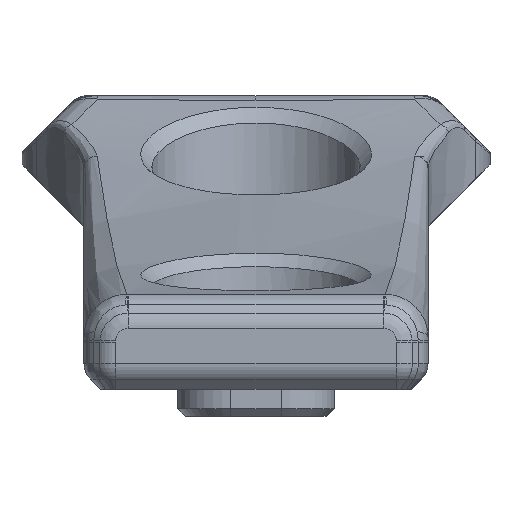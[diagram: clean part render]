
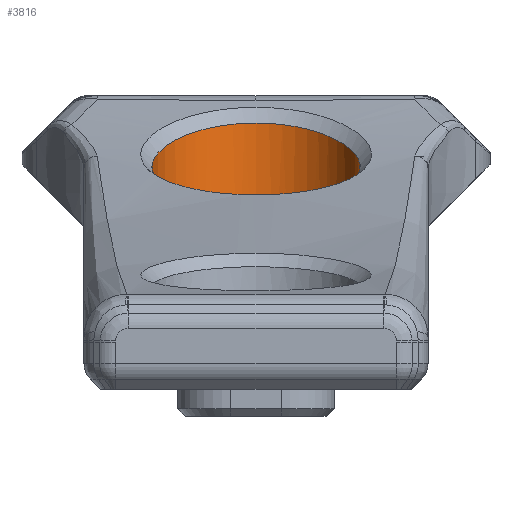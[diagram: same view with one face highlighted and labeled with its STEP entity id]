
A CAD part, front view. The second image highlights one B-rep face of the part: STEP entity #3816.
In plain terms, the highlighted cylindrical face has radius 4.65 mm (diameter 9.3 mm), a full revolution.
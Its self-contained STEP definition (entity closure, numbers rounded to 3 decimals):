
#304=CIRCLE('',#4113,4.65);
#429=FACE_OUTER_BOUND('',#678,.T.);
#678=EDGE_LOOP('',(#2908,#2909,#2910,#2911,#2912));
#931=LINE('',#6753,#1177);
#1177=VECTOR('',#4613,4.65);
#1433=B_SPLINE_CURVE_WITH_KNOTS('',3,(#6720,#6721,#6722,#6723,#6724,#6725,
#6726,#6727,#6728,#6729,#6730,#6731,#6732,#6733,#6734,#6735,#6736,#6737,
#6738,#6739),.UNSPECIFIED.,.F.,.F.,(4,1,1,1,1,1,1,1,1,1,1,1,1,1,1,1,1,4),
(0.,0.207,0.311,0.415,0.57,
0.622,0.829,0.968,1.244,1.313,
1.382,1.521,1.659,1.762,1.866,
2.022,2.073,2.155),.UNSPECIFIED.);
#1434=B_SPLINE_CURVE_WITH_KNOTS('',3,(#6740,#6741,#6742,#6743,#6744,#6745,
#6746,#6747,#6748,#6749),.UNSPECIFIED.,.F.,.F.,(4,1,1,1,1,1,1,4),(2.155,
2.281,2.488,2.566,2.592,2.696,
2.799,2.903),.UNSPECIFIED.);
#1711=VERTEX_POINT('',#6717);
#1712=VERTEX_POINT('',#6719);
#1713=VERTEX_POINT('',#6751);
#2141=EDGE_CURVE('',#1711,#1712,#1433,.T.);
#2142=EDGE_CURVE('',#1712,#1711,#1434,.T.);
#2143=EDGE_CURVE('',#1713,#1713,#304,.T.);
#2144=EDGE_CURVE('',#1713,#1712,#931,.T.);
#2908=ORIENTED_EDGE('',*,*,#2143,.T.);
#2909=ORIENTED_EDGE('',*,*,#2144,.T.);
#2910=ORIENTED_EDGE('',*,*,#2141,.F.);
#2911=ORIENTED_EDGE('',*,*,#2142,.F.);
#2912=ORIENTED_EDGE('',*,*,#2144,.F.);
#3699=CYLINDRICAL_SURFACE('',#4112,4.65);
#3816=ADVANCED_FACE('',(#429),#3699,.F.);
#4112=AXIS2_PLACEMENT_3D('',#6750,#4609,#4610);
#4113=AXIS2_PLACEMENT_3D('',#6752,#4611,#4612);
#4609=DIRECTION('center_axis',(0.,0.,1.));
#4610=DIRECTION('ref_axis',(1.,0.,0.));
#4611=DIRECTION('center_axis',(0.,0.,-1.));
#4612=DIRECTION('ref_axis',(1.,0.,0.));
#4613=DIRECTION('',(0.,0.,1.));
#6717=CARTESIAN_POINT('',(0.,38.65,11.102));
#6719=CARTESIAN_POINT('',(-4.651,33.998,9.158));
#6720=CARTESIAN_POINT('Ctrl Pts',(0.,38.65,11.102));
#6721=CARTESIAN_POINT('Ctrl Pts',(0.658,38.65,11.102));
#6722=CARTESIAN_POINT('Ctrl Pts',(1.717,38.423,10.996));
#6723=CARTESIAN_POINT('Ctrl Pts',(2.883,37.691,10.668));
#6724=CARTESIAN_POINT('Ctrl Pts',(3.701,36.904,10.325));
#6725=CARTESIAN_POINT('Ctrl Pts',(4.242,36.007,9.949));
#6726=CARTESIAN_POINT('Ctrl Pts',(4.657,34.705,9.426));
#6727=CARTESIAN_POINT('Ctrl Pts',(4.731,33.442,8.942));
#6728=CARTESIAN_POINT('Ctrl Pts',(4.041,31.371,8.202));
#6729=CARTESIAN_POINT('Ctrl Pts',(2.857,30.163,7.806));
#6730=CARTESIAN_POINT('Ctrl Pts',(1.461,29.563,7.614));
#6731=CARTESIAN_POINT('Ctrl Pts',(0.482,29.332,7.541));
#6732=CARTESIAN_POINT('Ctrl Pts',(-0.723,29.327,7.539));
#6733=CARTESIAN_POINT('Ctrl Pts',(-2.074,29.764,7.677));
#6734=CARTESIAN_POINT('Ctrl Pts',(-3.084,30.469,7.907));
#6735=CARTESIAN_POINT('Ctrl Pts',(-3.906,31.364,8.207));
#6736=CARTESIAN_POINT('Ctrl Pts',(-4.397,32.351,8.55));
#6737=CARTESIAN_POINT('Ctrl Pts',(-4.611,33.303,8.897));
#6738=CARTESIAN_POINT('Ctrl Pts',(-4.65,33.736,9.059));
#6739=CARTESIAN_POINT('Ctrl Pts',(-4.651,33.998,9.158));
#6740=CARTESIAN_POINT('Ctrl Pts',(-4.651,33.998,9.158));
#6741=CARTESIAN_POINT('Ctrl Pts',(-4.653,34.402,9.311));
#6742=CARTESIAN_POINT('Ctrl Pts',(-4.516,35.456,9.72));
#6743=CARTESIAN_POINT('Ctrl Pts',(-3.868,36.72,10.245));
#6744=CARTESIAN_POINT('Ctrl Pts',(-3.174,37.411,10.546));
#6745=CARTESIAN_POINT('Ctrl Pts',(-2.669,37.828,10.729));
#6746=CARTESIAN_POINT('Ctrl Pts',(-2.006,38.239,10.913));
#6747=CARTESIAN_POINT('Ctrl Pts',(-1.013,38.578,11.069));
#6748=CARTESIAN_POINT('Ctrl Pts',(-0.329,38.65,11.102));
#6749=CARTESIAN_POINT('Ctrl Pts',(0.,38.65,11.102));
#6750=CARTESIAN_POINT('Origin',(0.,34.,-2.));
#6751=CARTESIAN_POINT('',(-4.65,34.,2.8));
#6752=CARTESIAN_POINT('Origin',(0.,34.,2.8));
#6753=CARTESIAN_POINT('',(-4.65,34.,-2.));
